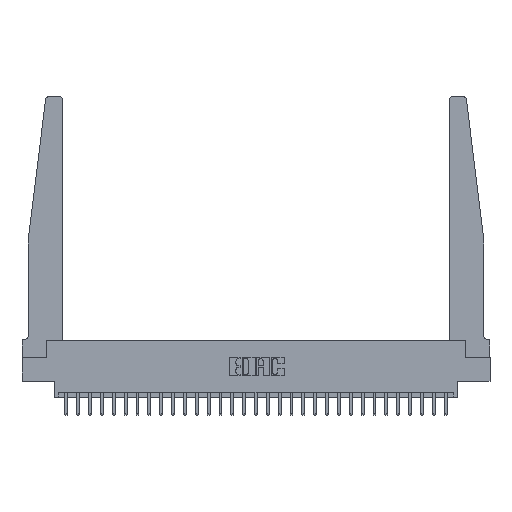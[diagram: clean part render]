
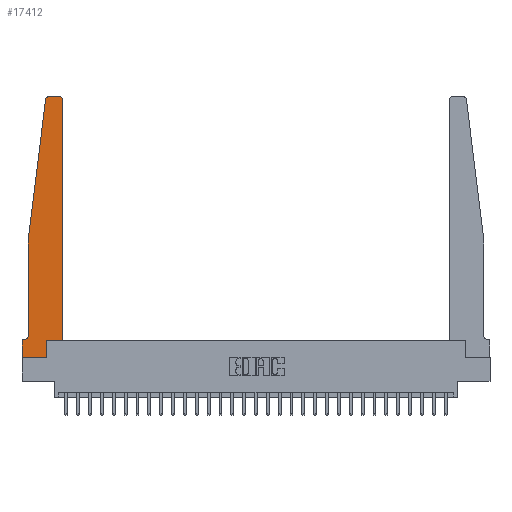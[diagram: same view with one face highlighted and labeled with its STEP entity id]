
A CAD part, top view. The second image highlights one B-rep face of the part: STEP entity #17412.
In plain terms, the highlighted planar face has unit normal (0, 0, 1).
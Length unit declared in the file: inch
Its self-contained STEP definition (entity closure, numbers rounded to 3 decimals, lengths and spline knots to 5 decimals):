
#60 = LINE ( 'NONE', #26892, #16903 ) ;
#269 = DIRECTION ( 'NONE',  ( 0., 0., 1. ) ) ;
#391 = ORIENTED_EDGE ( 'NONE', *, *, #13507, .T. ) ;
#669 = EDGE_CURVE ( 'NONE', #16130, #21827, #2028, .T. ) ;
#1062 = ORIENTED_EDGE ( 'NONE', *, *, #2700, .T. ) ;
#1104 = VERTEX_POINT ( 'NONE', #25303 ) ;
#1214 = DIRECTION ( 'NONE',  ( 0., -1., 0. ) ) ;
#1349 = LINE ( 'NONE', #10132, #12989 ) ;
#1609 = DIRECTION ( 'NONE',  ( -1., 0., 0. ) ) ;
#1936 = CARTESIAN_POINT ( 'NONE',  ( 0.425, 2.72, 0.37 ) ) ;
#2028 = LINE ( 'NONE', #3456, #24265 ) ;
#2300 = LINE ( 'NONE', #7166, #23882 ) ;
#2404 = VERTEX_POINT ( 'NONE', #19111 ) ;
#2632 = ORIENTED_EDGE ( 'NONE', *, *, #22807, .T. ) ;
#2700 = EDGE_CURVE ( 'NONE', #26441, #14378, #1349, .T. ) ;
#3175 = DIRECTION ( 'NONE',  ( 0., 1., 0. ) ) ;
#3456 = CARTESIAN_POINT ( 'NONE',  ( 0.2605, 0.18, 0.37 ) ) ;
#4296 = VECTOR ( 'NONE', #15321, 39.37008 ) ;
#4535 = ORIENTED_EDGE ( 'NONE', *, *, #13885, .T. ) ;
#5314 = VERTEX_POINT ( 'NONE', #1936 ) ;
#5394 = ORIENTED_EDGE ( 'NONE', *, *, #26054, .T. ) ;
#5975 = VERTEX_POINT ( 'NONE', #26681 ) ;
#6747 = FACE_OUTER_BOUND ( 'NONE', #15153, .T. ) ;
#6771 = CARTESIAN_POINT ( 'NONE',  ( 0.425, 0.18, 0.37 ) ) ;
#6807 = AXIS2_PLACEMENT_3D ( 'NONE', #13429, #269, #15645 ) ;
#7166 = CARTESIAN_POINT ( 'NONE',  ( 0.065, 1.25, 0.37 ) ) ;
#7649 = CARTESIAN_POINT ( 'NONE',  ( 0., 0.1875, 0.37 ) ) ;
#8131 = CARTESIAN_POINT ( 'NONE',  ( 0.425, 0.18, 0.37 ) ) ;
#8252 = VECTOR ( 'NONE', #17736, 39.37008 ) ;
#10050 = EDGE_CURVE ( 'NONE', #14485, #5314, #25266, .T. ) ;
#10132 = CARTESIAN_POINT ( 'NONE',  ( 0.065, 0.1875, 0.37 ) ) ;
#10630 = DIRECTION ( 'NONE',  ( -1., 0., 0. ) ) ;
#10820 = CARTESIAN_POINT ( 'NONE',  ( 0.395, 2.72, 0.37 ) ) ;
#11320 = EDGE_CURVE ( 'NONE', #2404, #15915, #26456, .T. ) ;
#11864 = EDGE_CURVE ( 'NONE', #5975, #2404, #2300, .T. ) ;
#11968 = CARTESIAN_POINT ( 'NONE',  ( 0.015, 0.2375, 0.37 ) ) ;
#12322 = DIRECTION ( 'NONE',  ( 1., 0., 0. ) ) ;
#12949 = ORIENTED_EDGE ( 'NONE', *, *, #11320, .T. ) ;
#12989 = VECTOR ( 'NONE', #10630, 39.37008 ) ;
#13014 = DIRECTION ( 'NONE',  ( 1., 0., 0. ) ) ;
#13146 = VECTOR ( 'NONE', #25197, 39.37008 ) ;
#13429 = CARTESIAN_POINT ( 'NONE',  ( 0.27653, 2.72, 0.37 ) ) ;
#13507 = EDGE_CURVE ( 'NONE', #5314, #1104, #20535, .T. ) ;
#13885 = EDGE_CURVE ( 'NONE', #14378, #26007, #60, .T. ) ;
#14176 = DIRECTION ( 'NONE',  ( -1., 0., 0. ) ) ;
#14378 = VERTEX_POINT ( 'NONE', #7649 ) ;
#14485 = VERTEX_POINT ( 'NONE', #16613 ) ;
#14981 = EDGE_CURVE ( 'NONE', #15915, #26441, #26504, .T. ) ;
#15153 = EDGE_LOOP ( 'NONE', ( #5394, #16625, #27588, #12949, #19463, #1062, #4535, #2632, #16731, #27517, #18819, #391 ) ) ;
#15321 = DIRECTION ( 'NONE',  ( 1., 0., 0. ) ) ;
#15645 = DIRECTION ( 'NONE',  ( 1., 0., 0. ) ) ;
#15915 = VERTEX_POINT ( 'NONE', #21509 ) ;
#15954 = CARTESIAN_POINT ( 'NONE',  ( 0.2605, 0., 0.37 ) ) ;
#16130 = VERTEX_POINT ( 'NONE', #15954 ) ;
#16459 = EDGE_CURVE ( 'NONE', #22146, #5975, #23283, .T. ) ;
#16613 = CARTESIAN_POINT ( 'NONE',  ( 0.425, 0.18, 0.37 ) ) ;
#16625 = ORIENTED_EDGE ( 'NONE', *, *, #16459, .T. ) ;
#16731 = ORIENTED_EDGE ( 'NONE', *, *, #669, .T. ) ;
#16861 = AXIS2_PLACEMENT_3D ( 'NONE', #11968, #26746, #14176 ) ;
#16903 = VECTOR ( 'NONE', #1214, 39.37008 ) ;
#17412 = ADVANCED_FACE ( 'NONE', ( #6747 ), #22969, .T. ) ;
#17736 = DIRECTION ( 'NONE',  ( 0., 1., 0. ) ) ;
#18469 = VECTOR ( 'NONE', #1609, 39.37008 ) ;
#18776 = CARTESIAN_POINT ( 'NONE',  ( 0., 0.1875, 0.37 ) ) ;
#18779 = EDGE_CURVE ( 'NONE', #21827, #14485, #18912, .T. ) ;
#18819 = ORIENTED_EDGE ( 'NONE', *, *, #10050, .T. ) ;
#18912 = LINE ( 'NONE', #8131, #13146 ) ;
#19042 = CARTESIAN_POINT ( 'NONE',  ( 0.25, 2.75, 0.37 ) ) ;
#19111 = CARTESIAN_POINT ( 'NONE',  ( 0.065, 1.25, 0.37 ) ) ;
#19463 = ORIENTED_EDGE ( 'NONE', *, *, #14981, .T. ) ;
#19955 = CARTESIAN_POINT ( 'NONE',  ( 0.015, 0.1875, 0.37 ) ) ;
#20126 = CARTESIAN_POINT ( 'NONE',  ( 0.2605, 0.18, 0.37 ) ) ;
#20149 = CARTESIAN_POINT ( 'NONE',  ( 0.065, 1.25, 0.37 ) ) ;
#20535 = CIRCLE ( 'NONE', #23684, 0.03 ) ;
#20916 = LINE ( 'NONE', #21718, #4296 ) ;
#21509 = CARTESIAN_POINT ( 'NONE',  ( 0.065, 0.2375, 0.37 ) ) ;
#21718 = CARTESIAN_POINT ( 'NONE',  ( 0., 0., 0.37 ) ) ;
#21827 = VERTEX_POINT ( 'NONE', #20126 ) ;
#22146 = VERTEX_POINT ( 'NONE', #23495 ) ;
#22807 = EDGE_CURVE ( 'NONE', #26007, #16130, #20916, .T. ) ;
#22969 = PLANE ( 'NONE',  #25769 ) ;
#23283 = CIRCLE ( 'NONE', #6807, 0.03 ) ;
#23495 = CARTESIAN_POINT ( 'NONE',  ( 0.27653, 2.75, 0.37 ) ) ;
#23684 = AXIS2_PLACEMENT_3D ( 'NONE', #10820, #25666, #13014 ) ;
#23882 = VECTOR ( 'NONE', #24303, 39.37008 ) ;
#24265 = VECTOR ( 'NONE', #3175, 39.37008 ) ;
#24303 = DIRECTION ( 'NONE',  ( -0.122, -0.992, 0. ) ) ;
#24658 = LINE ( 'NONE', #19042, #18469 ) ;
#24678 = DIRECTION ( 'NONE',  ( 0., -1., 0. ) ) ;
#25042 = DIRECTION ( 'NONE',  ( 0., 0., 1. ) ) ;
#25197 = DIRECTION ( 'NONE',  ( 1., 0., 0. ) ) ;
#25266 = LINE ( 'NONE', #6771, #8252 ) ;
#25303 = CARTESIAN_POINT ( 'NONE',  ( 0.395, 2.75, 0.37 ) ) ;
#25666 = DIRECTION ( 'NONE',  ( 0., 0., 1. ) ) ;
#25769 = AXIS2_PLACEMENT_3D ( 'NONE', #18776, #25042, #12322 ) ;
#25806 = VECTOR ( 'NONE', #24678, 39.37008 ) ;
#26007 = VERTEX_POINT ( 'NONE', #27153 ) ;
#26054 = EDGE_CURVE ( 'NONE', #1104, #22146, #24658, .T. ) ;
#26441 = VERTEX_POINT ( 'NONE', #19955 ) ;
#26456 = LINE ( 'NONE', #20149, #25806 ) ;
#26504 = CIRCLE ( 'NONE', #16861, 0.05 ) ;
#26681 = CARTESIAN_POINT ( 'NONE',  ( 0.24675, 2.72367, 0.37 ) ) ;
#26746 = DIRECTION ( 'NONE',  ( 0., 0., -1. ) ) ;
#26892 = CARTESIAN_POINT ( 'NONE',  ( 0., 0., 0.37 ) ) ;
#27153 = CARTESIAN_POINT ( 'NONE',  ( 0., 0., 0.37 ) ) ;
#27517 = ORIENTED_EDGE ( 'NONE', *, *, #18779, .T. ) ;
#27588 = ORIENTED_EDGE ( 'NONE', *, *, #11864, .T. ) ;
